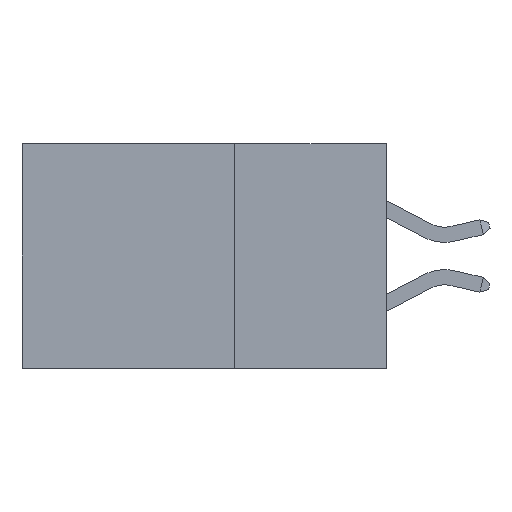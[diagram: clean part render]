
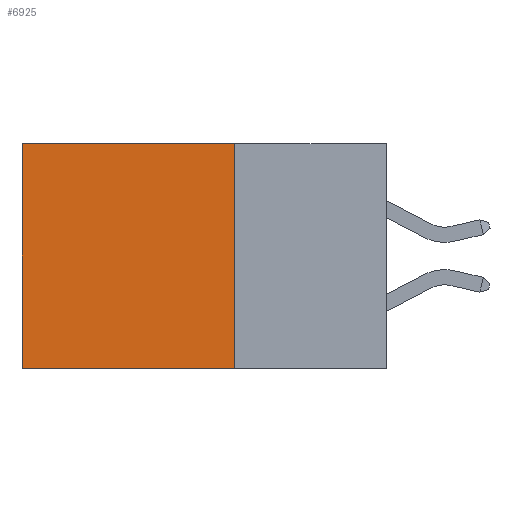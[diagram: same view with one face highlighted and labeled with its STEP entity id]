
A CAD part, left-side view. The second image highlights one B-rep face of the part: STEP entity #6925.
In plain terms, the highlighted planar face has unit normal (-1, 0, 0).
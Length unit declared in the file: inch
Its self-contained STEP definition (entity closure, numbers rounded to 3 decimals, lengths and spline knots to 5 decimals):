
#32 = AXIS2_PLACEMENT_3D ( 'NONE', #13801, #7511, #7490 ) ;
#403 = VERTEX_POINT ( 'NONE', #2844 ) ;
#405 = VERTEX_POINT ( 'NONE', #11316 ) ;
#2259 = VECTOR ( 'NONE', #15670, 39.37008 ) ;
#2581 = EDGE_CURVE ( 'NONE', #15726, #405, #12264, .T. ) ;
#2844 = CARTESIAN_POINT ( 'NONE',  ( 0.298, 0.6, -0.37 ) ) ;
#3487 = VERTEX_POINT ( 'NONE', #5004 ) ;
#3628 = VECTOR ( 'NONE', #5121, 39.37008 ) ;
#4198 = DIRECTION ( 'NONE',  ( 0., 0., -1. ) ) ;
#4592 = VECTOR ( 'NONE', #4198, 39.37008 ) ;
#5004 = CARTESIAN_POINT ( 'NONE',  ( 0.298, 0.25, -0.37 ) ) ;
#5121 = DIRECTION ( 'NONE',  ( 0., 1., 0. ) ) ;
#5847 = FACE_OUTER_BOUND ( 'NONE', #9323, .T. ) ;
#6912 = ORIENTED_EDGE ( 'NONE', *, *, #2581, .T. ) ;
#6925 = ADVANCED_FACE ( 'NONE', ( #5847 ), #10511, .F. ) ;
#7490 = DIRECTION ( 'NONE',  ( 0., 0., -1. ) ) ;
#7492 = ORIENTED_EDGE ( 'NONE', *, *, #9794, .T. ) ;
#7511 = DIRECTION ( 'NONE',  ( 1., 0., 0. ) ) ;
#7686 = LINE ( 'NONE', #8829, #3628 ) ;
#8319 = CARTESIAN_POINT ( 'NONE',  ( 0.298, 0.6, 0. ) ) ;
#8477 = VECTOR ( 'NONE', #13126, 39.37008 ) ;
#8829 = CARTESIAN_POINT ( 'NONE',  ( 0.298, 0.25, -0.37 ) ) ;
#9323 = EDGE_LOOP ( 'NONE', ( #7492, #9515, #9912, #6912 ) ) ;
#9515 = ORIENTED_EDGE ( 'NONE', *, *, #10381, .F. ) ;
#9794 = EDGE_CURVE ( 'NONE', #405, #403, #15389, .T. ) ;
#9912 = ORIENTED_EDGE ( 'NONE', *, *, #10551, .F. ) ;
#10084 = CARTESIAN_POINT ( 'NONE',  ( 0.298, 0.25, 0. ) ) ;
#10381 = EDGE_CURVE ( 'NONE', #3487, #403, #7686, .T. ) ;
#10511 = PLANE ( 'NONE',  #32 ) ;
#10551 = EDGE_CURVE ( 'NONE', #15726, #3487, #10881, .T. ) ;
#10881 = LINE ( 'NONE', #11728, #4592 ) ;
#11316 = CARTESIAN_POINT ( 'NONE',  ( 0.298, 0.6, 0. ) ) ;
#11728 = CARTESIAN_POINT ( 'NONE',  ( 0.298, 0.25, 0. ) ) ;
#12264 = LINE ( 'NONE', #10084, #8477 ) ;
#13126 = DIRECTION ( 'NONE',  ( 0., 1., 0. ) ) ;
#13801 = CARTESIAN_POINT ( 'NONE',  ( 0.298, 0.25, 0. ) ) ;
#15389 = LINE ( 'NONE', #8319, #2259 ) ;
#15670 = DIRECTION ( 'NONE',  ( 0., 0., -1. ) ) ;
#15726 = VERTEX_POINT ( 'NONE', #15789 ) ;
#15789 = CARTESIAN_POINT ( 'NONE',  ( 0.298, 0.25, 0. ) ) ;
